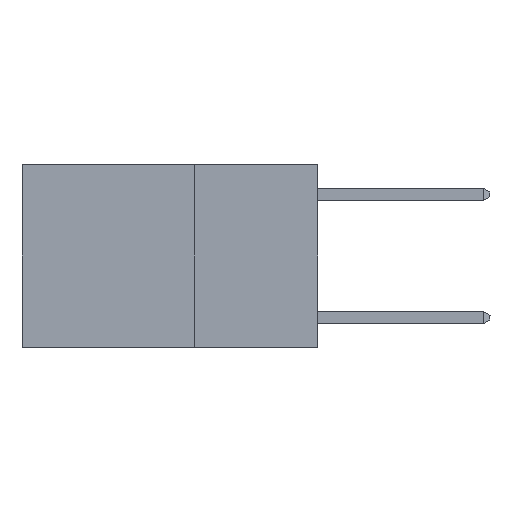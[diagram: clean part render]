
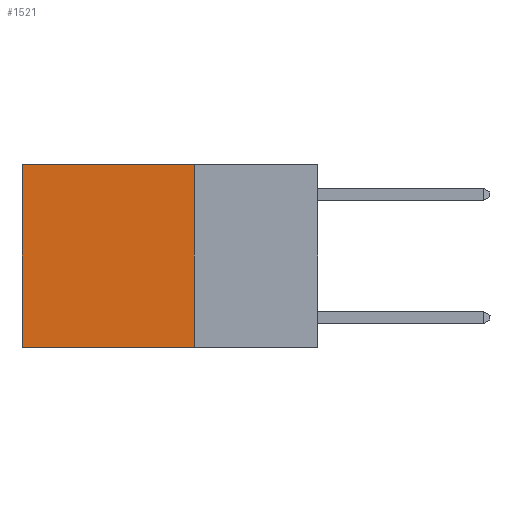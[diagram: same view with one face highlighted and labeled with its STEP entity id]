
A CAD part, left-side view. The second image highlights one B-rep face of the part: STEP entity #1521.
In plain terms, the highlighted planar face has unit normal (-1, 0, 0).
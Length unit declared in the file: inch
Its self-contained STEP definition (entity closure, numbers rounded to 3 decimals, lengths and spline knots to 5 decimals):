
#548 = VERTEX_POINT ( 'NONE', #30811 ) ;
#1236 = LINE ( 'NONE', #5455, #20242 ) ;
#1384 = VECTOR ( 'NONE', #23577, 39.37008 ) ;
#1521 = ADVANCED_FACE ( 'NONE', ( #30688 ), #19709, .F. ) ;
#2469 = CARTESIAN_POINT ( 'NONE',  ( 0.2625, 0.25, 0. ) ) ;
#4370 = ORIENTED_EDGE ( 'NONE', *, *, #5672, .F. ) ;
#5019 = DIRECTION ( 'NONE',  ( 0., 0., -1. ) ) ;
#5157 = EDGE_CURVE ( 'NONE', #29902, #548, #1236, .T. ) ;
#5455 = CARTESIAN_POINT ( 'NONE',  ( 0.2625, 0.25, 0. ) ) ;
#5672 = EDGE_CURVE ( 'NONE', #29902, #19253, #7912, .T. ) ;
#6116 = ORIENTED_EDGE ( 'NONE', *, *, #5157, .T. ) ;
#7912 = LINE ( 'NONE', #12202, #20213 ) ;
#7986 = DIRECTION ( 'NONE',  ( 0., 1., 0. ) ) ;
#8300 = EDGE_CURVE ( 'NONE', #548, #13596, #9204, .T. ) ;
#9204 = LINE ( 'NONE', #19107, #27807 ) ;
#9462 = AXIS2_PLACEMENT_3D ( 'NONE', #2469, #19811, #5019 ) ;
#10298 = CARTESIAN_POINT ( 'NONE',  ( 0.2625, 0.6, -0.37 ) ) ;
#12202 = CARTESIAN_POINT ( 'NONE',  ( 0.2625, 0.25, 0. ) ) ;
#13596 = VERTEX_POINT ( 'NONE', #10298 ) ;
#16652 = DIRECTION ( 'NONE',  ( 0., 0., -1. ) ) ;
#17230 = DIRECTION ( 'NONE',  ( 0., 0., -1. ) ) ;
#19003 = ORIENTED_EDGE ( 'NONE', *, *, #8300, .T. ) ;
#19107 = CARTESIAN_POINT ( 'NONE',  ( 0.2625, 0.6, 0. ) ) ;
#19253 = VERTEX_POINT ( 'NONE', #30919 ) ;
#19709 = PLANE ( 'NONE',  #9462 ) ;
#19811 = DIRECTION ( 'NONE',  ( 1., 0., 0. ) ) ;
#20213 = VECTOR ( 'NONE', #17230, 39.37008 ) ;
#20242 = VECTOR ( 'NONE', #7986, 39.37008 ) ;
#21114 = LINE ( 'NONE', #21174, #1384 ) ;
#21174 = CARTESIAN_POINT ( 'NONE',  ( 0.2625, 0.25, -0.37 ) ) ;
#23103 = CARTESIAN_POINT ( 'NONE',  ( 0.2625, 0.25, 0. ) ) ;
#23577 = DIRECTION ( 'NONE',  ( 0., 1., 0. ) ) ;
#27807 = VECTOR ( 'NONE', #16652, 39.37008 ) ;
#28191 = EDGE_LOOP ( 'NONE', ( #19003, #30132, #4370, #6116 ) ) ;
#29902 = VERTEX_POINT ( 'NONE', #23103 ) ;
#30132 = ORIENTED_EDGE ( 'NONE', *, *, #30700, .F. ) ;
#30688 = FACE_OUTER_BOUND ( 'NONE', #28191, .T. ) ;
#30700 = EDGE_CURVE ( 'NONE', #19253, #13596, #21114, .T. ) ;
#30811 = CARTESIAN_POINT ( 'NONE',  ( 0.2625, 0.6, 0. ) ) ;
#30919 = CARTESIAN_POINT ( 'NONE',  ( 0.2625, 0.25, -0.37 ) ) ;
